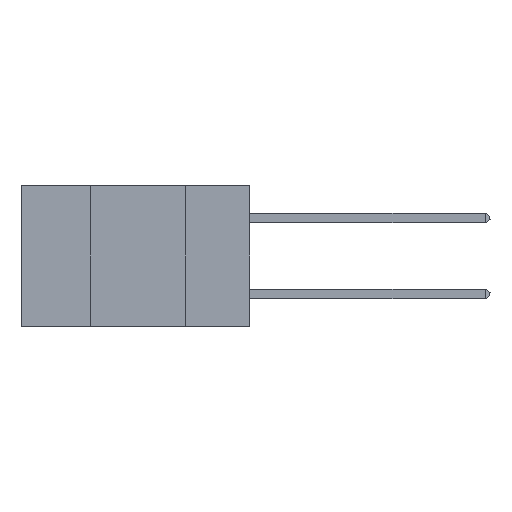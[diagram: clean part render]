
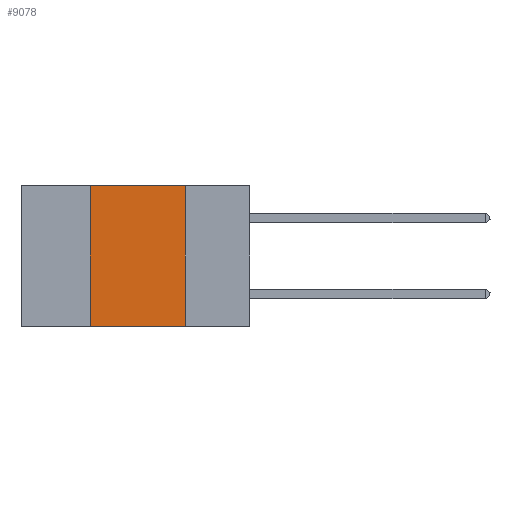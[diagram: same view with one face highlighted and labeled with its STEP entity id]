
A CAD part, left-side view. The second image highlights one B-rep face of the part: STEP entity #9078.
In plain terms, the highlighted planar face has unit normal (-1, 0, 0).
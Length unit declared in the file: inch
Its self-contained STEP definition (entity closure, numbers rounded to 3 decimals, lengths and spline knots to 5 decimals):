
#3553 = ORIENTED_EDGE ( 'NONE', *, *, #20574, .T. ) ;
#5051 = CARTESIAN_POINT ( 'NONE',  ( 0., 0.17, 0. ) ) ;
#5646 = CARTESIAN_POINT ( 'NONE',  ( 0., 0.6, -0.37 ) ) ;
#7936 = DIRECTION ( 'NONE',  ( 0., 0., -1. ) ) ;
#8008 = VECTOR ( 'NONE', #38778, 39.37008 ) ;
#8216 = DIRECTION ( 'NONE',  ( 0., 0., 1. ) ) ;
#8419 = CARTESIAN_POINT ( 'NONE',  ( 0., 0.6, 0. ) ) ;
#9078 = ADVANCED_FACE ( 'NONE', ( #9841 ), #37907, .F. ) ;
#9409 = ORIENTED_EDGE ( 'NONE', *, *, #14837, .F. ) ;
#9841 = FACE_OUTER_BOUND ( 'NONE', #28007, .T. ) ;
#10361 = VERTEX_POINT ( 'NONE', #23304 ) ;
#11485 = ORIENTED_EDGE ( 'NONE', *, *, #11744, .F. ) ;
#11744 = EDGE_CURVE ( 'NONE', #17555, #27111, #28427, .T. ) ;
#11750 = VECTOR ( 'NONE', #23092, 39.37008 ) ;
#14837 = EDGE_CURVE ( 'NONE', #23401, #10361, #19687, .T. ) ;
#16742 = LINE ( 'NONE', #8419, #30888 ) ;
#17442 = CARTESIAN_POINT ( 'NONE',  ( 0., 0.17, 0. ) ) ;
#17521 = EDGE_CURVE ( 'NONE', #27111, #23401, #16742, .T. ) ;
#17555 = VERTEX_POINT ( 'NONE', #32609 ) ;
#19687 = LINE ( 'NONE', #5051, #11750 ) ;
#19885 = CARTESIAN_POINT ( 'NONE',  ( 0., 0.6, 0. ) ) ;
#20574 = EDGE_CURVE ( 'NONE', #17555, #10361, #23079, .T. ) ;
#23079 = LINE ( 'NONE', #5646, #8008 ) ;
#23092 = DIRECTION ( 'NONE',  ( 0., 0., -1. ) ) ;
#23304 = CARTESIAN_POINT ( 'NONE',  ( 0., 0.17, -0.37 ) ) ;
#23401 = VERTEX_POINT ( 'NONE', #17442 ) ;
#24714 = CARTESIAN_POINT ( 'NONE',  ( 0., 0.42, 0. ) ) ;
#25995 = DIRECTION ( 'NONE',  ( 1., 0., 0. ) ) ;
#27111 = VERTEX_POINT ( 'NONE', #24714 ) ;
#27487 = VECTOR ( 'NONE', #8216, 39.37008 ) ;
#28007 = EDGE_LOOP ( 'NONE', ( #9409, #34273, #11485, #3553 ) ) ;
#28427 = LINE ( 'NONE', #29284, #27487 ) ;
#29284 = CARTESIAN_POINT ( 'NONE',  ( 0., 0.42, 0. ) ) ;
#30888 = VECTOR ( 'NONE', #35491, 39.37008 ) ;
#32609 = CARTESIAN_POINT ( 'NONE',  ( 0., 0.42, -0.37 ) ) ;
#33834 = AXIS2_PLACEMENT_3D ( 'NONE', #19885, #25995, #7936 ) ;
#34273 = ORIENTED_EDGE ( 'NONE', *, *, #17521, .F. ) ;
#35491 = DIRECTION ( 'NONE',  ( 0., -1., 0. ) ) ;
#37907 = PLANE ( 'NONE',  #33834 ) ;
#38778 = DIRECTION ( 'NONE',  ( 0., -1., 0. ) ) ;
